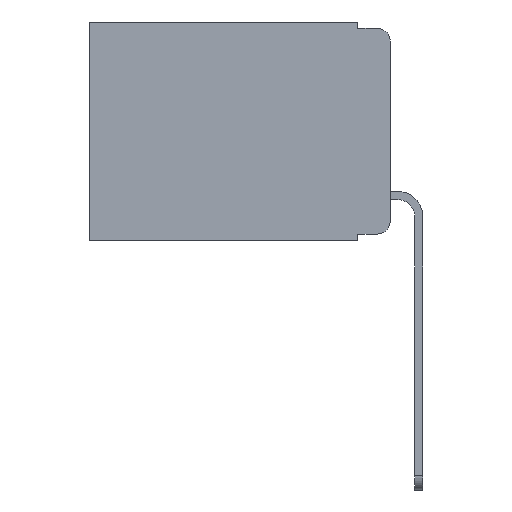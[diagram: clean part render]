
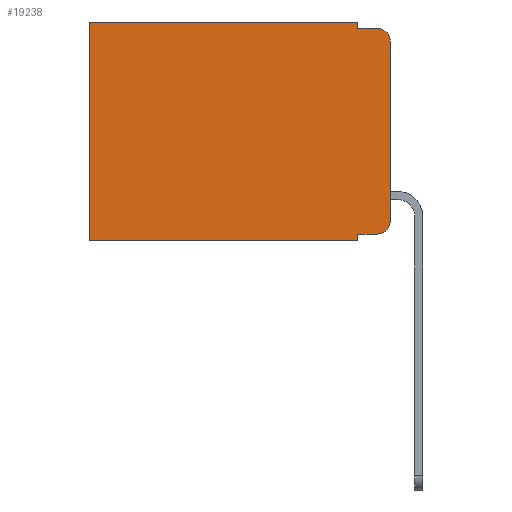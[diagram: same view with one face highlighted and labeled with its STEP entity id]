
A CAD part, left-side view. The second image highlights one B-rep face of the part: STEP entity #19238.
In plain terms, the highlighted planar face has unit normal (-1, 0, 0).
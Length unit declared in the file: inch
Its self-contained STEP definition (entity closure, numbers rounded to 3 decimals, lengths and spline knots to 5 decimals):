
#925 = VERTEX_POINT ( 'NONE', #2698 ) ;
#1063 = DIRECTION ( 'NONE',  ( 0., 0., -1. ) ) ;
#1476 = DIRECTION ( 'NONE',  ( 0., -1., 0. ) ) ;
#1542 = VECTOR ( 'NONE', #13396, 39.37008 ) ;
#1558 = AXIS2_PLACEMENT_3D ( 'NONE', #20451, #9147, #22262 ) ;
#1562 = ORIENTED_EDGE ( 'NONE', *, *, #17484, .F. ) ;
#1618 = CARTESIAN_POINT ( 'NONE',  ( 0.298, 0.473, 0. ) ) ;
#2153 = VERTEX_POINT ( 'NONE', #17781 ) ;
#2173 = DIRECTION ( 'NONE',  ( 0., 0., -1. ) ) ;
#2300 = DIRECTION ( 'NONE',  ( 0., 1., 0. ) ) ;
#2547 = LINE ( 'NONE', #21967, #12412 ) ;
#2698 = CARTESIAN_POINT ( 'NONE',  ( 0.298, 0.473, 0. ) ) ;
#3120 = DIRECTION ( 'NONE',  ( 0., 0., -1. ) ) ;
#3292 = DIRECTION ( 'NONE',  ( 0., 1., 0. ) ) ;
#3924 = VECTOR ( 'NONE', #24285, 39.37008 ) ;
#3973 = VECTOR ( 'NONE', #11576, 39.37008 ) ;
#3991 = EDGE_CURVE ( 'NONE', #23428, #20746, #2547, .T. ) ;
#4078 = CIRCLE ( 'NONE', #1558, 0.02 ) ;
#4835 = CARTESIAN_POINT ( 'NONE',  ( 0.298, 0.02, -0.313 ) ) ;
#4876 = ORIENTED_EDGE ( 'NONE', *, *, #14739, .F. ) ;
#5187 = EDGE_CURVE ( 'NONE', #5323, #15768, #11469, .T. ) ;
#5323 = VERTEX_POINT ( 'NONE', #17921 ) ;
#5324 = CARTESIAN_POINT ( 'NONE',  ( 0.298, 0., 0. ) ) ;
#5609 = VERTEX_POINT ( 'NONE', #6603 ) ;
#5618 = VERTEX_POINT ( 'NONE', #24807 ) ;
#6386 = VECTOR ( 'NONE', #3120, 39.37008 ) ;
#6403 = ORIENTED_EDGE ( 'NONE', *, *, #16664, .F. ) ;
#6603 = CARTESIAN_POINT ( 'NONE',  ( 0.298, 0.051, -0.01 ) ) ;
#6802 = DIRECTION ( 'NONE',  ( 0., 0., -1. ) ) ;
#6890 = VECTOR ( 'NONE', #2173, 39.37008 ) ;
#7132 = CARTESIAN_POINT ( 'NONE',  ( 0.298, 0., -0.03 ) ) ;
#7422 = CIRCLE ( 'NONE', #17952, 0.02 ) ;
#8571 = LINE ( 'NONE', #9612, #3973 ) ;
#9147 = DIRECTION ( 'NONE',  ( -1., 0., 0. ) ) ;
#9612 = CARTESIAN_POINT ( 'NONE',  ( 0.298, 0.051, -0.01 ) ) ;
#10178 = VERTEX_POINT ( 'NONE', #13039 ) ;
#11469 = LINE ( 'NONE', #19263, #21923 ) ;
#11576 = DIRECTION ( 'NONE',  ( 0., -1., 0. ) ) ;
#12412 = VECTOR ( 'NONE', #2300, 39.37008 ) ;
#12670 = LINE ( 'NONE', #15782, #6890 ) ;
#12889 = DIRECTION ( 'NONE',  ( 1., 0., 0. ) ) ;
#13039 = CARTESIAN_POINT ( 'NONE',  ( 0.298, 0.02, -0.01 ) ) ;
#13396 = DIRECTION ( 'NONE',  ( 0., 0., -1. ) ) ;
#14303 = ORIENTED_EDGE ( 'NONE', *, *, #20732, .T. ) ;
#14729 = ORIENTED_EDGE ( 'NONE', *, *, #20258, .T. ) ;
#14736 = CARTESIAN_POINT ( 'NONE',  ( 0.298, 0.051, 0. ) ) ;
#14739 = EDGE_CURVE ( 'NONE', #2153, #5609, #20923, .T. ) ;
#15076 = CARTESIAN_POINT ( 'NONE',  ( 0.298, 0., 0. ) ) ;
#15768 = VERTEX_POINT ( 'NONE', #17652 ) ;
#15782 = CARTESIAN_POINT ( 'NONE',  ( 0.298, 0.051, 0. ) ) ;
#16353 = CARTESIAN_POINT ( 'NONE',  ( 0.298, 0.473, -0.343 ) ) ;
#16534 = AXIS2_PLACEMENT_3D ( 'NONE', #23959, #12889, #1063 ) ;
#16560 = PLANE ( 'NONE',  #16534 ) ;
#16588 = ORIENTED_EDGE ( 'NONE', *, *, #19326, .T. ) ;
#16664 = EDGE_CURVE ( 'NONE', #5609, #10178, #8571, .T. ) ;
#17484 = EDGE_CURVE ( 'NONE', #23990, #5618, #18609, .T. ) ;
#17621 = LINE ( 'NONE', #1618, #1542 ) ;
#17652 = CARTESIAN_POINT ( 'NONE',  ( 0.298, 0.02, -0.333 ) ) ;
#17781 = CARTESIAN_POINT ( 'NONE',  ( 0.298, 0.051, 0. ) ) ;
#17921 = CARTESIAN_POINT ( 'NONE',  ( 0.298, 0.051, -0.333 ) ) ;
#17952 = AXIS2_PLACEMENT_3D ( 'NONE', #4835, #18226, #6802 ) ;
#18226 = DIRECTION ( 'NONE',  ( -1., 0., 0. ) ) ;
#18609 = LINE ( 'NONE', #15076, #3924 ) ;
#18657 = CARTESIAN_POINT ( 'NONE',  ( 0.298, 0.051, -0.343 ) ) ;
#19238 = ADVANCED_FACE ( 'NONE', ( #22821 ), #16560, .F. ) ;
#19263 = CARTESIAN_POINT ( 'NONE',  ( 0.298, 0.051, -0.333 ) ) ;
#19302 = ORIENTED_EDGE ( 'NONE', *, *, #23713, .F. ) ;
#19326 = EDGE_CURVE ( 'NONE', #2153, #925, #21674, .T. ) ;
#19486 = ORIENTED_EDGE ( 'NONE', *, *, #24134, .T. ) ;
#19856 = ORIENTED_EDGE ( 'NONE', *, *, #5187, .T. ) ;
#20137 = ORIENTED_EDGE ( 'NONE', *, *, #3991, .F. ) ;
#20258 = EDGE_CURVE ( 'NONE', #23990, #10178, #4078, .T. ) ;
#20451 = CARTESIAN_POINT ( 'NONE',  ( 0.298, 0.02, -0.03 ) ) ;
#20553 = VECTOR ( 'NONE', #3292, 39.37008 ) ;
#20732 = EDGE_CURVE ( 'NONE', #15768, #5618, #7422, .T. ) ;
#20746 = VERTEX_POINT ( 'NONE', #16353 ) ;
#20923 = LINE ( 'NONE', #14736, #6386 ) ;
#21221 = EDGE_LOOP ( 'NONE', ( #1562, #14729, #6403, #4876, #16588, #19486, #20137, #19302, #19856, #14303 ) ) ;
#21674 = LINE ( 'NONE', #5324, #20553 ) ;
#21923 = VECTOR ( 'NONE', #1476, 39.37008 ) ;
#21967 = CARTESIAN_POINT ( 'NONE',  ( 0.298, 0., -0.343 ) ) ;
#22262 = DIRECTION ( 'NONE',  ( 0., 0., -1. ) ) ;
#22821 = FACE_OUTER_BOUND ( 'NONE', #21221, .T. ) ;
#23428 = VERTEX_POINT ( 'NONE', #18657 ) ;
#23713 = EDGE_CURVE ( 'NONE', #5323, #23428, #12670, .T. ) ;
#23959 = CARTESIAN_POINT ( 'NONE',  ( 0.298, 0., 0. ) ) ;
#23990 = VERTEX_POINT ( 'NONE', #7132 ) ;
#24134 = EDGE_CURVE ( 'NONE', #925, #20746, #17621, .T. ) ;
#24285 = DIRECTION ( 'NONE',  ( 0., 0., -1. ) ) ;
#24807 = CARTESIAN_POINT ( 'NONE',  ( 0.298, 0., -0.313 ) ) ;
